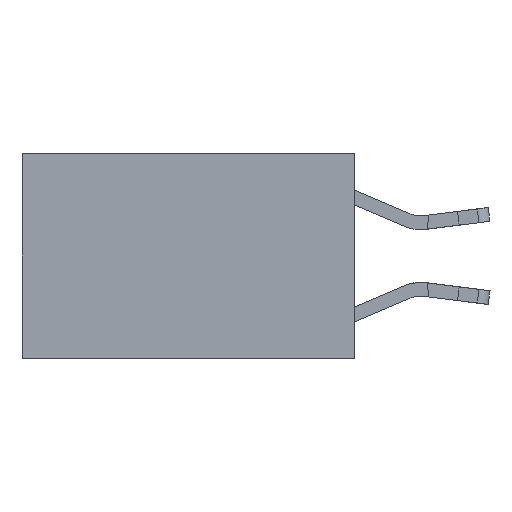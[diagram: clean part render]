
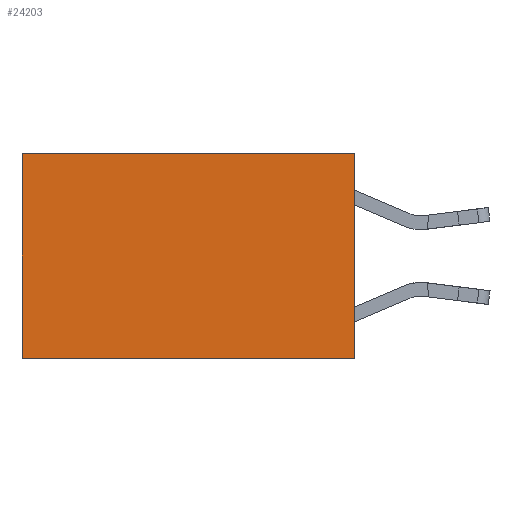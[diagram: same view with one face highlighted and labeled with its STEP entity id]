
A CAD part, left-side view. The second image highlights one B-rep face of the part: STEP entity #24203.
In plain terms, the highlighted planar face has unit normal (-1, 0, 0).
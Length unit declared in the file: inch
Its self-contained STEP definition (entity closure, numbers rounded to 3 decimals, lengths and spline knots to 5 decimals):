
#161 = DIRECTION ( 'NONE',  ( 0., 1., 0. ) ) ;
#890 = LINE ( 'NONE', #15710, #21991 ) ;
#1188 = CARTESIAN_POINT ( 'NONE',  ( 0.2625, 0., -0.37 ) ) ;
#2220 = EDGE_CURVE ( 'NONE', #23471, #23971, #14190, .T. ) ;
#3362 = VECTOR ( 'NONE', #161, 39.37008 ) ;
#4310 = CARTESIAN_POINT ( 'NONE',  ( 0.2625, 0.6, 0. ) ) ;
#6227 = FACE_OUTER_BOUND ( 'NONE', #7677, .T. ) ;
#7677 = EDGE_LOOP ( 'NONE', ( #22647, #19911, #8758, #11877 ) ) ;
#8758 = ORIENTED_EDGE ( 'NONE', *, *, #13541, .F. ) ;
#10230 = VECTOR ( 'NONE', #17864, 39.37008 ) ;
#11754 = CARTESIAN_POINT ( 'NONE',  ( 0.2625, 0., 0. ) ) ;
#11877 = ORIENTED_EDGE ( 'NONE', *, *, #12968, .T. ) ;
#11931 = VECTOR ( 'NONE', #22563, 39.37008 ) ;
#12128 = CARTESIAN_POINT ( 'NONE',  ( 0.2625, 0., 0. ) ) ;
#12968 = EDGE_CURVE ( 'NONE', #14312, #14789, #16240, .T. ) ;
#13541 = EDGE_CURVE ( 'NONE', #14312, #23471, #890, .T. ) ;
#14175 = PLANE ( 'NONE',  #24807 ) ;
#14190 = LINE ( 'NONE', #24674, #3362 ) ;
#14312 = VERTEX_POINT ( 'NONE', #22857 ) ;
#14789 = VERTEX_POINT ( 'NONE', #4310 ) ;
#15710 = CARTESIAN_POINT ( 'NONE',  ( 0.2625, 0., 0. ) ) ;
#16208 = DIRECTION ( 'NONE',  ( 0., 0., -1. ) ) ;
#16240 = LINE ( 'NONE', #11754, #10230 ) ;
#16454 = CARTESIAN_POINT ( 'NONE',  ( 0.2625, 0.6, 0. ) ) ;
#17743 = DIRECTION ( 'NONE',  ( 0., 0., -1. ) ) ;
#17864 = DIRECTION ( 'NONE',  ( 0., 1., 0. ) ) ;
#19911 = ORIENTED_EDGE ( 'NONE', *, *, #2220, .F. ) ;
#20398 = EDGE_CURVE ( 'NONE', #14789, #23971, #22789, .T. ) ;
#21991 = VECTOR ( 'NONE', #17743, 39.37008 ) ;
#22317 = DIRECTION ( 'NONE',  ( 1., 0., 0. ) ) ;
#22563 = DIRECTION ( 'NONE',  ( 0., 0., -1. ) ) ;
#22647 = ORIENTED_EDGE ( 'NONE', *, *, #20398, .T. ) ;
#22789 = LINE ( 'NONE', #16454, #11931 ) ;
#22857 = CARTESIAN_POINT ( 'NONE',  ( 0.2625, 0., 0. ) ) ;
#23471 = VERTEX_POINT ( 'NONE', #1188 ) ;
#23585 = CARTESIAN_POINT ( 'NONE',  ( 0.2625, 0.6, -0.37 ) ) ;
#23971 = VERTEX_POINT ( 'NONE', #23585 ) ;
#24203 = ADVANCED_FACE ( 'NONE', ( #6227 ), #14175, .F. ) ;
#24674 = CARTESIAN_POINT ( 'NONE',  ( 0.2625, 0., -0.37 ) ) ;
#24807 = AXIS2_PLACEMENT_3D ( 'NONE', #12128, #22317, #16208 ) ;
